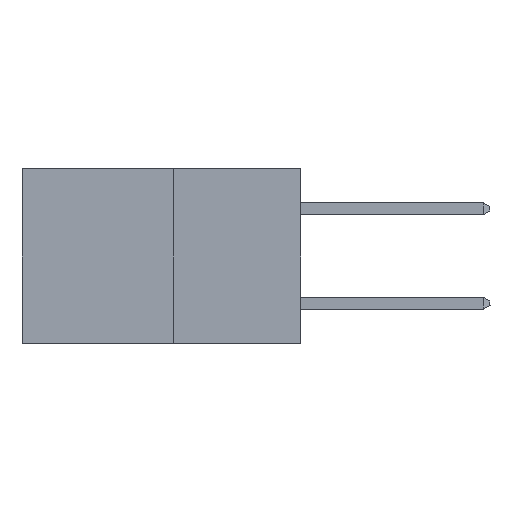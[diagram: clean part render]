
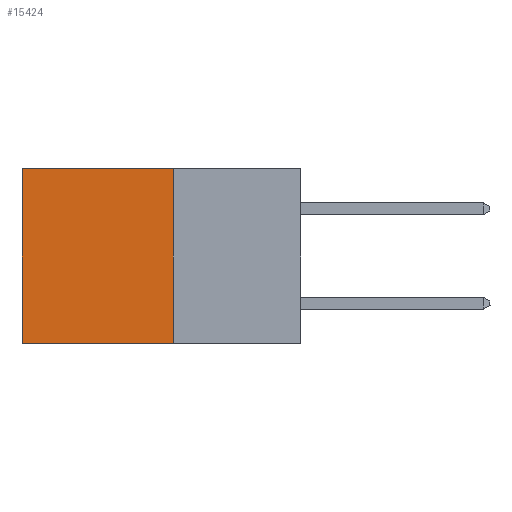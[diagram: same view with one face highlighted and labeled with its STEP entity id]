
A CAD part, left-side view. The second image highlights one B-rep face of the part: STEP entity #15424.
In plain terms, the highlighted planar face has unit normal (-1, 0, 0).
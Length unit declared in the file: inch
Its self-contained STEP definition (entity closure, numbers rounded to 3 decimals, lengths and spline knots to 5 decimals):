
#508 = VECTOR ( 'NONE', #5854, 39.37008 ) ;
#630 = EDGE_LOOP ( 'NONE', ( #17519, #2834, #8625, #9492 ) ) ;
#767 = VECTOR ( 'NONE', #15558, 39.37008 ) ;
#2355 = PLANE ( 'NONE',  #18424 ) ;
#2782 = VECTOR ( 'NONE', #5983, 39.37008 ) ;
#2834 = ORIENTED_EDGE ( 'NONE', *, *, #3014, .F. ) ;
#3014 = EDGE_CURVE ( 'NONE', #20655, #19857, #12168, .T. ) ;
#3568 = FACE_OUTER_BOUND ( 'NONE', #630, .T. ) ;
#4075 = DIRECTION ( 'NONE',  ( 0., 0., -1. ) ) ;
#4129 = CARTESIAN_POINT ( 'NONE',  ( 0.277, 0.59, -0.37 ) ) ;
#5215 = CARTESIAN_POINT ( 'NONE',  ( 0.277, 0.27, 0. ) ) ;
#5854 = DIRECTION ( 'NONE',  ( 0., 0., -1. ) ) ;
#5983 = DIRECTION ( 'NONE',  ( 0., 0., -1. ) ) ;
#8625 = ORIENTED_EDGE ( 'NONE', *, *, #14772, .F. ) ;
#9492 = ORIENTED_EDGE ( 'NONE', *, *, #11505, .T. ) ;
#9665 = LINE ( 'NONE', #4129, #508 ) ;
#9907 = LINE ( 'NONE', #5215, #767 ) ;
#11505 = EDGE_CURVE ( 'NONE', #18171, #12030, #9907, .T. ) ;
#12030 = VERTEX_POINT ( 'NONE', #18545 ) ;
#12168 = LINE ( 'NONE', #13030, #14302 ) ;
#13030 = CARTESIAN_POINT ( 'NONE',  ( 0.277, 0.27, -0.37 ) ) ;
#13732 = CARTESIAN_POINT ( 'NONE',  ( 0.277, 0.27, 0. ) ) ;
#14302 = VECTOR ( 'NONE', #19619, 39.37008 ) ;
#14396 = DIRECTION ( 'NONE',  ( 1., 0., 0. ) ) ;
#14509 = CARTESIAN_POINT ( 'NONE',  ( 0.277, 0.59, -0.37 ) ) ;
#14772 = EDGE_CURVE ( 'NONE', #18171, #20655, #15974, .T. ) ;
#15424 = ADVANCED_FACE ( 'NONE', ( #3568 ), #2355, .F. ) ;
#15558 = DIRECTION ( 'NONE',  ( 0., 1., 0. ) ) ;
#15974 = LINE ( 'NONE', #16323, #2782 ) ;
#16068 = CARTESIAN_POINT ( 'NONE',  ( 0.277, 0.27, -0.37 ) ) ;
#16323 = CARTESIAN_POINT ( 'NONE',  ( 0.277, 0.27, -0.37 ) ) ;
#17128 = EDGE_CURVE ( 'NONE', #12030, #19857, #9665, .T. ) ;
#17519 = ORIENTED_EDGE ( 'NONE', *, *, #17128, .T. ) ;
#18024 = CARTESIAN_POINT ( 'NONE',  ( 0.277, 0.27, -0.37 ) ) ;
#18171 = VERTEX_POINT ( 'NONE', #13732 ) ;
#18424 = AXIS2_PLACEMENT_3D ( 'NONE', #16068, #14396, #4075 ) ;
#18545 = CARTESIAN_POINT ( 'NONE',  ( 0.277, 0.59, 0. ) ) ;
#19619 = DIRECTION ( 'NONE',  ( 0., 1., 0. ) ) ;
#19857 = VERTEX_POINT ( 'NONE', #14509 ) ;
#20655 = VERTEX_POINT ( 'NONE', #18024 ) ;
